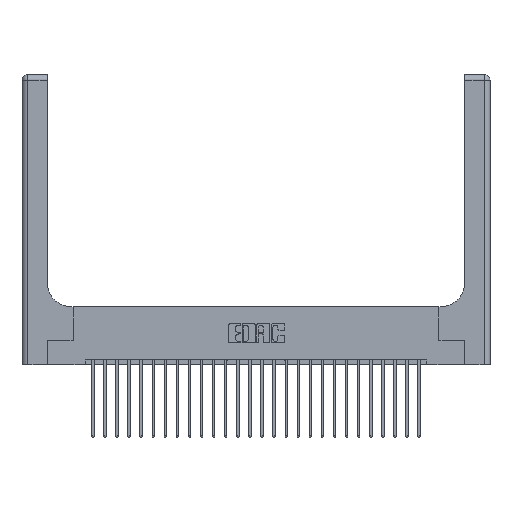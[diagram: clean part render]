
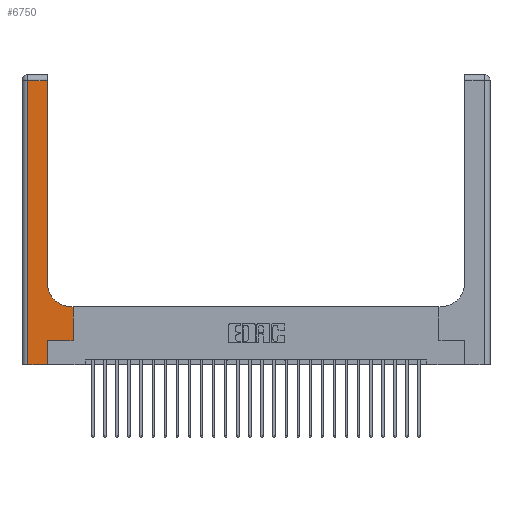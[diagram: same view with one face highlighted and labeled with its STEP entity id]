
A CAD part, top view. The second image highlights one B-rep face of the part: STEP entity #6750.
In plain terms, the highlighted planar face has unit normal (0, 0, 1).
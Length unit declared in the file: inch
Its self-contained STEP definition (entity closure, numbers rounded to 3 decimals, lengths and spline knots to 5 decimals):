
#234 = EDGE_LOOP ( 'NONE', ( #17229, #21861, #5566, #13437, #20830, #16545, #14752, #2479, #16179 ) ) ;
#624 = CARTESIAN_POINT ( 'NONE',  ( 0.265, 0., 0.37 ) ) ;
#678 = CARTESIAN_POINT ( 'NONE',  ( 0.26, 3., 0.37 ) ) ;
#1242 = VECTOR ( 'NONE', #8480, 39.37008 ) ;
#1731 = CARTESIAN_POINT ( 'NONE',  ( 0.26, 0.6, 0.37 ) ) ;
#1942 = DIRECTION ( 'NONE',  ( 1., 0., 0. ) ) ;
#2304 = VECTOR ( 'NONE', #6250, 39.37008 ) ;
#2464 = CIRCLE ( 'NONE', #14835, 0.25 ) ;
#2479 = ORIENTED_EDGE ( 'NONE', *, *, #5676, .T. ) ;
#3452 = CARTESIAN_POINT ( 'NONE',  ( 0.06, 3., 0.37 ) ) ;
#3596 = EDGE_CURVE ( 'NONE', #12137, #19512, #14292, .T. ) ;
#3858 = VECTOR ( 'NONE', #17590, 39.37008 ) ;
#3891 = LINE ( 'NONE', #9530, #18921 ) ;
#3902 = DIRECTION ( 'NONE',  ( 0., 0., -1. ) ) ;
#3935 = CARTESIAN_POINT ( 'NONE',  ( 0., 2.94, 0.37 ) ) ;
#4239 = VERTEX_POINT ( 'NONE', #14067 ) ;
#5394 = VERTEX_POINT ( 'NONE', #20092 ) ;
#5428 = DIRECTION ( 'NONE',  ( 0., -1., 0. ) ) ;
#5566 = ORIENTED_EDGE ( 'NONE', *, *, #24810, .T. ) ;
#5676 = EDGE_CURVE ( 'NONE', #19512, #14640, #17572, .T. ) ;
#6250 = DIRECTION ( 'NONE',  ( 0., 1., 0. ) ) ;
#6645 = EDGE_CURVE ( 'NONE', #14569, #24358, #11684, .T. ) ;
#6750 = ADVANCED_FACE ( 'NONE', ( #7392 ), #6771, .F. ) ;
#6771 = PLANE ( 'NONE',  #10046 ) ;
#6953 = VECTOR ( 'NONE', #5428, 39.37008 ) ;
#7036 = EDGE_CURVE ( 'NONE', #14640, #14569, #2464, .T. ) ;
#7238 = DIRECTION ( 'NONE',  ( 1., 0., 0. ) ) ;
#7392 = FACE_OUTER_BOUND ( 'NONE', #234, .T. ) ;
#7849 = EDGE_CURVE ( 'NONE', #22668, #5394, #16216, .T. ) ;
#8129 = VECTOR ( 'NONE', #7238, 39.37008 ) ;
#8253 = VECTOR ( 'NONE', #16613, 39.37008 ) ;
#8480 = DIRECTION ( 'NONE',  ( 0., 1., 0. ) ) ;
#8700 = CARTESIAN_POINT ( 'NONE',  ( 0.26, 0.85, 0.37 ) ) ;
#8732 = DIRECTION ( 'NONE',  ( 0., 0., -1. ) ) ;
#8874 = VERTEX_POINT ( 'NONE', #17923 ) ;
#9085 = LINE ( 'NONE', #3935, #3858 ) ;
#9530 = CARTESIAN_POINT ( 'NONE',  ( 0.265, 0.25, 0.37 ) ) ;
#9951 = EDGE_CURVE ( 'NONE', #5394, #12137, #3891, .T. ) ;
#10046 = AXIS2_PLACEMENT_3D ( 'NONE', #24147, #8732, #10368 ) ;
#10368 = DIRECTION ( 'NONE',  ( -1., 0., 0. ) ) ;
#10835 = CARTESIAN_POINT ( 'NONE',  ( 0.528, 0.25, 0.37 ) ) ;
#11684 = LINE ( 'NONE', #678, #1242 ) ;
#12002 = CARTESIAN_POINT ( 'NONE',  ( 0.26, 2.94, 0.37 ) ) ;
#12137 = VERTEX_POINT ( 'NONE', #10835 ) ;
#12179 = LINE ( 'NONE', #3452, #6953 ) ;
#13437 = ORIENTED_EDGE ( 'NONE', *, *, #18177, .T. ) ;
#13985 = CARTESIAN_POINT ( 'NONE',  ( 0.51, 0.85, 0.37 ) ) ;
#14067 = CARTESIAN_POINT ( 'NONE',  ( 0.06, 0., 0.37 ) ) ;
#14292 = LINE ( 'NONE', #15786, #2304 ) ;
#14569 = VERTEX_POINT ( 'NONE', #8700 ) ;
#14640 = VERTEX_POINT ( 'NONE', #22397 ) ;
#14752 = ORIENTED_EDGE ( 'NONE', *, *, #3596, .T. ) ;
#14835 = AXIS2_PLACEMENT_3D ( 'NONE', #13985, #3902, #1942 ) ;
#15786 = CARTESIAN_POINT ( 'NONE',  ( 0.528, 0.25, 0.37 ) ) ;
#16179 = ORIENTED_EDGE ( 'NONE', *, *, #7036, .T. ) ;
#16216 = LINE ( 'NONE', #18749, #8253 ) ;
#16245 = CARTESIAN_POINT ( 'NONE',  ( 0., 0., 0.37 ) ) ;
#16545 = ORIENTED_EDGE ( 'NONE', *, *, #9951, .T. ) ;
#16613 = DIRECTION ( 'NONE',  ( 0., 1., 0. ) ) ;
#16844 = EDGE_CURVE ( 'NONE', #24358, #8874, #9085, .T. ) ;
#17229 = ORIENTED_EDGE ( 'NONE', *, *, #6645, .T. ) ;
#17441 = DIRECTION ( 'NONE',  ( -1., 0., 0. ) ) ;
#17572 = LINE ( 'NONE', #1731, #20302 ) ;
#17590 = DIRECTION ( 'NONE',  ( -1., 0., 0. ) ) ;
#17923 = CARTESIAN_POINT ( 'NONE',  ( 0.06, 2.94, 0.37 ) ) ;
#18177 = EDGE_CURVE ( 'NONE', #4239, #22668, #21609, .T. ) ;
#18749 = CARTESIAN_POINT ( 'NONE',  ( 0.265, 0., 0.37 ) ) ;
#18921 = VECTOR ( 'NONE', #25318, 39.37008 ) ;
#19512 = VERTEX_POINT ( 'NONE', #22234 ) ;
#20092 = CARTESIAN_POINT ( 'NONE',  ( 0.265, 0.25, 0.37 ) ) ;
#20302 = VECTOR ( 'NONE', #17441, 39.37008 ) ;
#20830 = ORIENTED_EDGE ( 'NONE', *, *, #7849, .T. ) ;
#21609 = LINE ( 'NONE', #16245, #8129 ) ;
#21861 = ORIENTED_EDGE ( 'NONE', *, *, #16844, .T. ) ;
#22234 = CARTESIAN_POINT ( 'NONE',  ( 0.528, 0.6, 0.37 ) ) ;
#22397 = CARTESIAN_POINT ( 'NONE',  ( 0.51, 0.6, 0.37 ) ) ;
#22668 = VERTEX_POINT ( 'NONE', #624 ) ;
#24147 = CARTESIAN_POINT ( 'NONE',  ( 0., 3., 0.37 ) ) ;
#24358 = VERTEX_POINT ( 'NONE', #12002 ) ;
#24810 = EDGE_CURVE ( 'NONE', #8874, #4239, #12179, .T. ) ;
#25318 = DIRECTION ( 'NONE',  ( 1., 0., 0. ) ) ;
